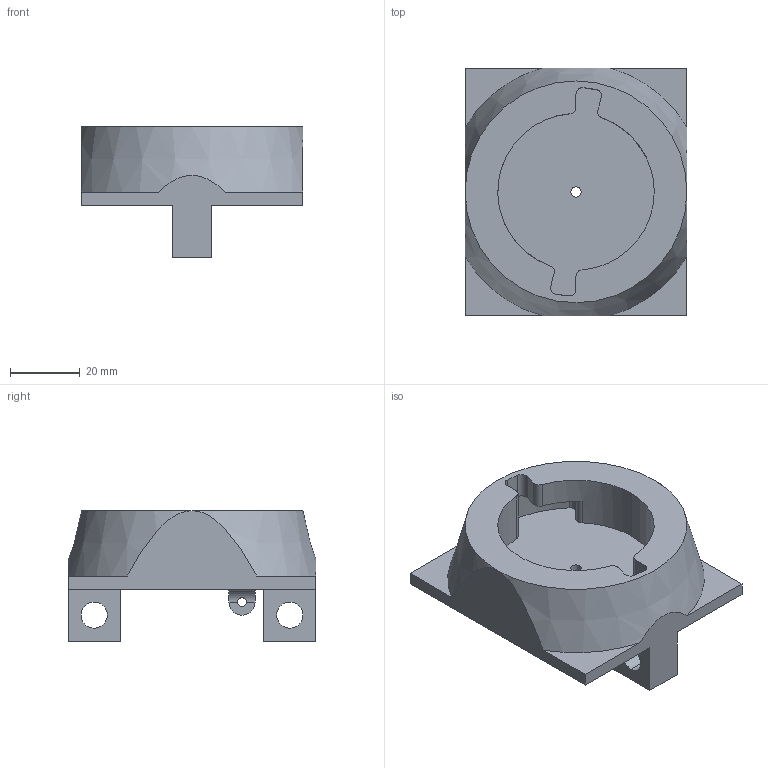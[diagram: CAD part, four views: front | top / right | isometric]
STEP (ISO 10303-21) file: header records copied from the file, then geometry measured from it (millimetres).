
FILE_DESCRIPTION (( 'STEP AP203' ), '1' );
FILE_NAME ('Nail_Block.STEP', '2013-09-22T12:20:54', ( '' ), ( '' ), 'SwSTEP 2.0', 'SolidWorks 2013', '' );
FILE_SCHEMA (( 'CONFIG_CONTROL_DESIGN' ));
Length unit declared in the file: millimetre
Products named in the file (1): Nail_Block
Bounding box: 63.75 x 71.25 x 37.5 mm (x, y, z)
Volume: 61765 mm3; surface area: 18544.9 mm2
Topology: 1 solids, 1 shells, 70 faces, 190 edges, 122 vertices
Faces by surface type: cylinder 33, plane 31, cone 4, torus 2
Entity records: 2465 total; most frequent: CARTESIAN_POINT 549, DIRECTION 404, ORIENTED_EDGE 380, EDGE_CURVE 190, AXIS2_PLACEMENT_3D 151, VERTEX_POINT 122, VECTOR 102, LINE 102
